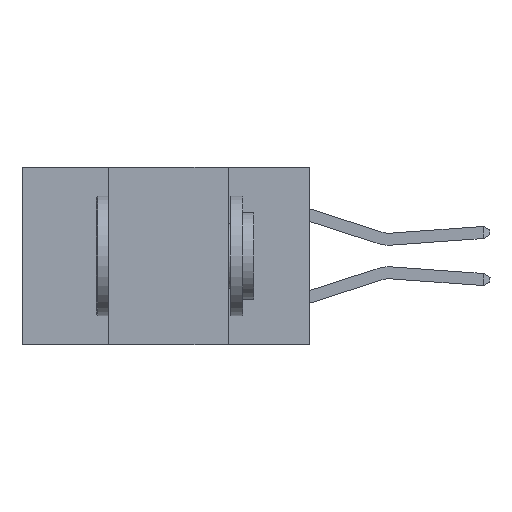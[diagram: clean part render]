
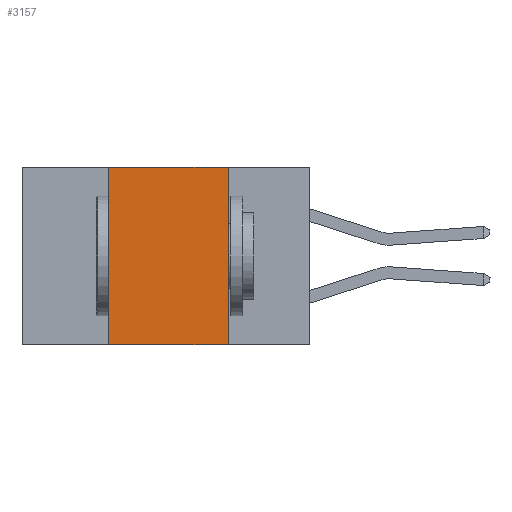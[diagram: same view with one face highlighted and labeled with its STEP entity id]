
A CAD part, left-side view. The second image highlights one B-rep face of the part: STEP entity #3157.
In plain terms, the highlighted planar face has unit normal (-1, 0, 0).
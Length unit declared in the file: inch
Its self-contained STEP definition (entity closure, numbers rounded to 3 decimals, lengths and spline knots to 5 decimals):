
#212 = VERTEX_POINT ( 'NONE', #10656 ) ;
#691 = DIRECTION ( 'NONE',  ( 1., 0., 0. ) ) ;
#921 = LINE ( 'NONE', #5644, #10649 ) ;
#1046 = ORIENTED_EDGE ( 'NONE', *, *, #1854, .T. ) ;
#1693 = AXIS2_PLACEMENT_3D ( 'NONE', #11268, #691, #7882 ) ;
#1708 = VECTOR ( 'NONE', #5913, 39.37008 ) ;
#1854 = EDGE_CURVE ( 'NONE', #212, #10318, #921, .T. ) ;
#2119 = DIRECTION ( 'NONE',  ( 0., -1., 0. ) ) ;
#2289 = LINE ( 'NONE', #10926, #1708 ) ;
#2519 = CARTESIAN_POINT ( 'NONE',  ( 0., 0.42, 0. ) ) ;
#2871 = CARTESIAN_POINT ( 'NONE',  ( 0., 0.17, 0. ) ) ;
#3157 = ADVANCED_FACE ( 'NONE', ( #9088 ), #3309, .F. ) ;
#3309 = PLANE ( 'NONE',  #1693 ) ;
#4093 = ORIENTED_EDGE ( 'NONE', *, *, #7782, .F. ) ;
#5038 = VECTOR ( 'NONE', #5067, 39.37008 ) ;
#5067 = DIRECTION ( 'NONE',  ( 0., 0., -1. ) ) ;
#5644 = CARTESIAN_POINT ( 'NONE',  ( 0., 0.6, -0.37 ) ) ;
#5913 = DIRECTION ( 'NONE',  ( 0., -1., 0. ) ) ;
#6056 = ORIENTED_EDGE ( 'NONE', *, *, #7010, .F. ) ;
#7010 = EDGE_CURVE ( 'NONE', #8982, #8849, #2289, .T. ) ;
#7592 = CARTESIAN_POINT ( 'NONE',  ( 0., 0.42, 0. ) ) ;
#7782 = EDGE_CURVE ( 'NONE', #8849, #10318, #10691, .T. ) ;
#7882 = DIRECTION ( 'NONE',  ( 0., 0., -1. ) ) ;
#8374 = CARTESIAN_POINT ( 'NONE',  ( 0., 0.17, -0.37 ) ) ;
#8849 = VERTEX_POINT ( 'NONE', #2871 ) ;
#8982 = VERTEX_POINT ( 'NONE', #2519 ) ;
#9088 = FACE_OUTER_BOUND ( 'NONE', #11134, .T. ) ;
#9430 = VECTOR ( 'NONE', #11161, 39.37008 ) ;
#9711 = CARTESIAN_POINT ( 'NONE',  ( 0., 0.17, 0. ) ) ;
#10318 = VERTEX_POINT ( 'NONE', #8374 ) ;
#10649 = VECTOR ( 'NONE', #2119, 39.37008 ) ;
#10656 = CARTESIAN_POINT ( 'NONE',  ( 0., 0.42, -0.37 ) ) ;
#10691 = LINE ( 'NONE', #9711, #5038 ) ;
#10926 = CARTESIAN_POINT ( 'NONE',  ( 0., 0.6, 0. ) ) ;
#11041 = EDGE_CURVE ( 'NONE', #212, #8982, #11202, .T. ) ;
#11134 = EDGE_LOOP ( 'NONE', ( #4093, #6056, #11285, #1046 ) ) ;
#11161 = DIRECTION ( 'NONE',  ( 0., 0., 1. ) ) ;
#11202 = LINE ( 'NONE', #7592, #9430 ) ;
#11268 = CARTESIAN_POINT ( 'NONE',  ( 0., 0.6, 0. ) ) ;
#11285 = ORIENTED_EDGE ( 'NONE', *, *, #11041, .F. ) ;
